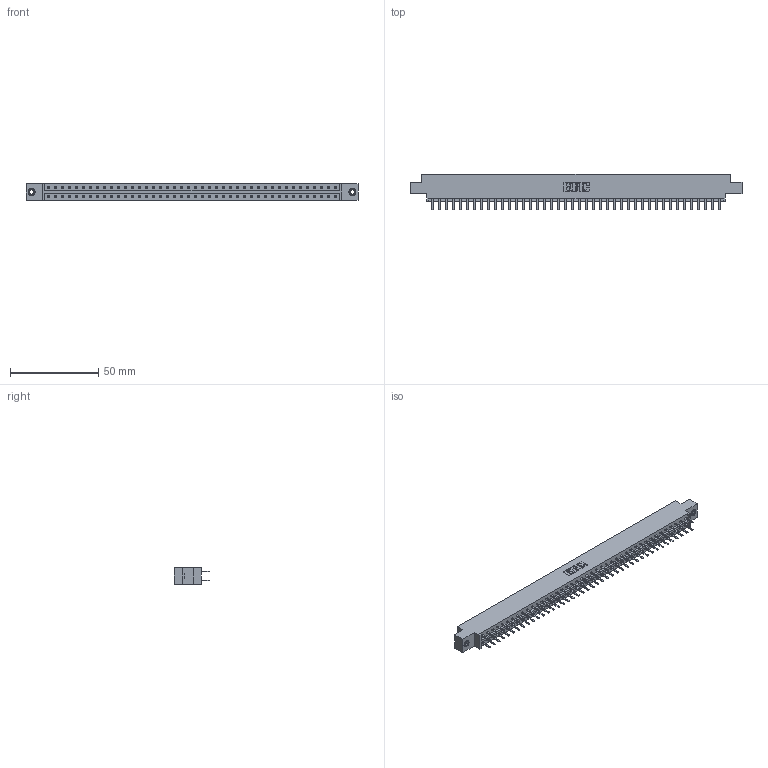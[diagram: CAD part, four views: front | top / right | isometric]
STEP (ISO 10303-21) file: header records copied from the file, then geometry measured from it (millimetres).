
FILE_DESCRIPTION (( 'STEP AP203' ), '1' );
FILE_NAME ('333-084-520-807.STEP', '2018-08-05T04:06:46', ( '' ), ( '' ), 'SwSTEP 2.0', 'SolidWorks 2016', '' );
FILE_SCHEMA (( 'CONFIG_CONTROL_DESIGN' ));
Length unit declared in the file: inch
Products named in the file (4): 345-250-001_345-250-005-103; 333-084-520-807; 333 Part_Offset - .156 Dia - TI; 345-292-001_345-293-120
Assembly tree (87 placements, depth 2):
  333-084-520-807
    333 Part_Offset - .156 Dia - TI
    345-292-001_345-293-120  x84
    345-250-001_345-250-005-103  x2
Bounding box: 187.96 x 20.02 x 9.4 mm (x, y, z)
Volume: 18911.4 mm3; surface area: 22515.1 mm2
Topology: 87 solids, 87 shells, 4882 faces, 14151 edges, 9202 vertices
Faces by surface type: plane 3298, cylinder 1568, cone 12, torus 4
Entity records: 28452 total; most frequent: CARTESIAN_POINT 4713, ORIENTED_EDGE 4630, DIRECTION 4045, EDGE_CURVE 2315, VECTOR 2163, LINE 2163, VERTEX_POINT 1536, AXIS2_PLACEMENT_3D 941
